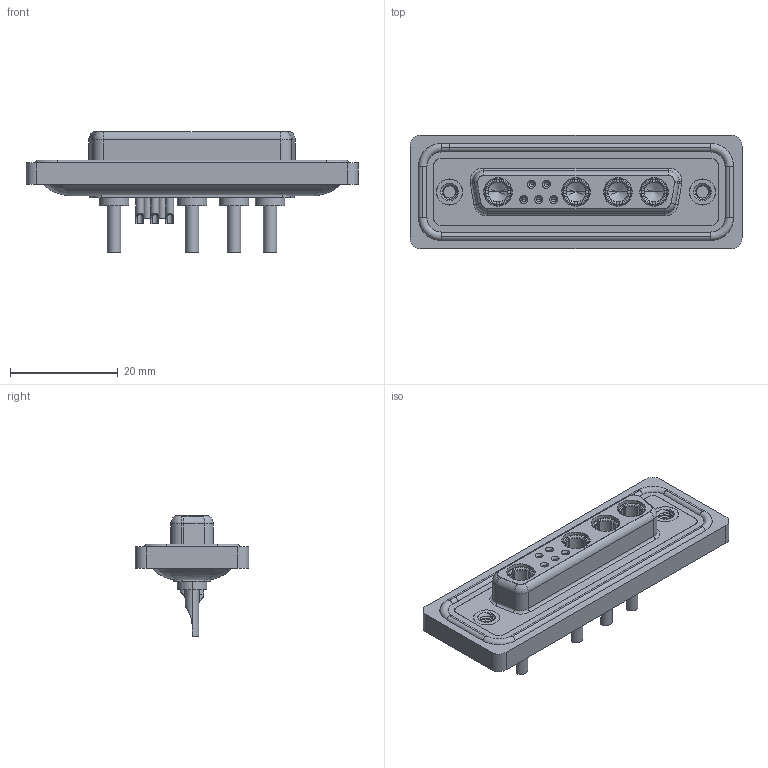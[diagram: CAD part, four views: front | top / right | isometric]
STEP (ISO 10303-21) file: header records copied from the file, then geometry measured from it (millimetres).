
FILE_DESCRIPTION (( 'STEP AP203' ), '1' );
FILE_NAME ('628W9W4-122-1N2.STEP', '2024-04-09T19:43:30', ( '' ), ( '' ), 'SwSTEP 2.0', 'SolidWorks 2023', '' );
FILE_SCHEMA (( 'CONFIG_CONTROL_DESIGN' ));
Length unit declared in the file: millimetre
Products named in the file (9): 628Combo Contact Row 1_22; 628Combo Shell Front_25 Contacts; 628Combo Contact Row 2_22; 628Combo Shell Rear_25 Contacts; 628W9W4-122-1N2; 628Combo Housing_9W4; Power Socket_10A SC; 628Combo Threaded Rivet_2; 628Combo Waterproof Housing_25 Contacts
Assembly tree (15 placements, depth 2):
  628W9W4-122-1N2
    628Combo Housing_9W4
    628Combo Waterproof Housing_25 Contacts
    628Combo Shell Front_25 Contacts
    628Combo Shell Rear_25 Contacts
    628Combo Threaded Rivet_2  x2
    628Combo Contact Row 1_22  x2
    628Combo Contact Row 2_22  x3
    Power Socket_10A SC  x4
Bounding box: 61.75 x 21.1 x 22.45 mm (x, y, z)
Volume: 8223.3 mm3; surface area: 13807.7 mm2
Topology: 20 solids, 20 shells, 977 faces, 2485 edges, 1562 vertices
Faces by surface type: cylinder 397, plane 314, torus 127, cone 125, bspline 14
Entity records: 20980 total; most frequent: CARTESIAN_POINT 5420, DIRECTION 3196, ORIENTED_EDGE 2936, EDGE_CURVE 1468, AXIS2_PLACEMENT_3D 1293, VERTEX_POINT 934, CIRCLE 687, EDGE_LOOP 672
